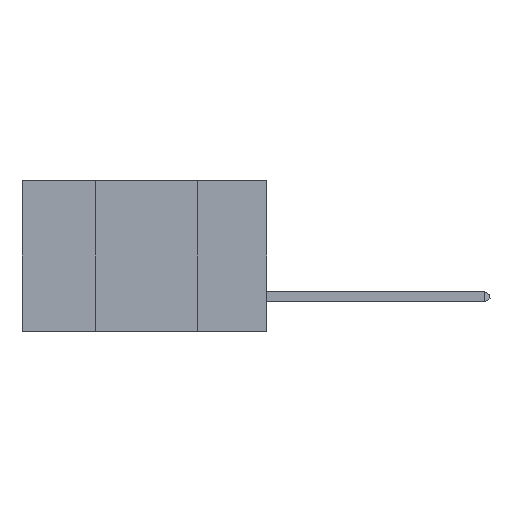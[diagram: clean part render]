
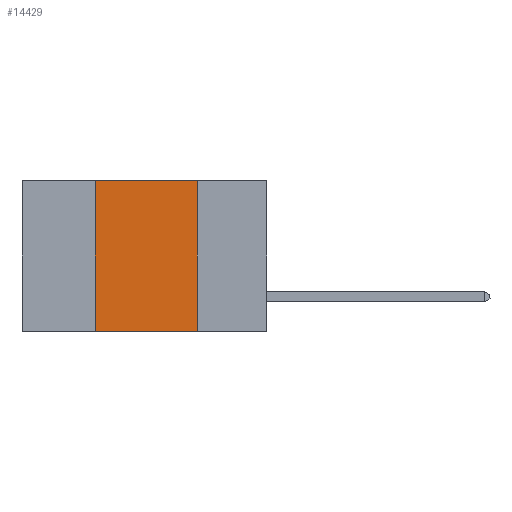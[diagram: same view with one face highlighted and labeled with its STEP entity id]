
A CAD part, left-side view. The second image highlights one B-rep face of the part: STEP entity #14429.
In plain terms, the highlighted planar face has unit normal (-1, 0, 0).
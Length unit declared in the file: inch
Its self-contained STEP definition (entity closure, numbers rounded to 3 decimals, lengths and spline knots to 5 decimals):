
#1192 = EDGE_CURVE ( 'NONE', #11467, #7550, #17679, .T. ) ;
#2617 = EDGE_CURVE ( 'NONE', #19219, #3082, #4087, .T. ) ;
#3082 = VERTEX_POINT ( 'NONE', #18073 ) ;
#3970 = ORIENTED_EDGE ( 'NONE', *, *, #1192, .F. ) ;
#4010 = ORIENTED_EDGE ( 'NONE', *, *, #2617, .F. ) ;
#4087 = LINE ( 'NONE', #20644, #19233 ) ;
#4941 = CARTESIAN_POINT ( 'NONE',  ( 0., 0.6, -0.37 ) ) ;
#5565 = EDGE_CURVE ( 'NONE', #3082, #11467, #14519, .T. ) ;
#7550 = VERTEX_POINT ( 'NONE', #15245 ) ;
#8149 = EDGE_CURVE ( 'NONE', #19219, #7550, #22864, .T. ) ;
#8182 = PLANE ( 'NONE',  #20640 ) ;
#8767 = DIRECTION ( 'NONE',  ( 0., -1., 0. ) ) ;
#10013 = ORIENTED_EDGE ( 'NONE', *, *, #5565, .F. ) ;
#11066 = FACE_OUTER_BOUND ( 'NONE', #22155, .T. ) ;
#11467 = VERTEX_POINT ( 'NONE', #24824 ) ;
#12265 = DIRECTION ( 'NONE',  ( 1., 0., 0. ) ) ;
#14363 = VECTOR ( 'NONE', #19330, 39.37008 ) ;
#14429 = ADVANCED_FACE ( 'NONE', ( #11066 ), #8182, .F. ) ;
#14519 = LINE ( 'NONE', #19071, #24931 ) ;
#15245 = CARTESIAN_POINT ( 'NONE',  ( 0., 0.17, -0.37 ) ) ;
#15873 = CARTESIAN_POINT ( 'NONE',  ( 0., 0.17, 0. ) ) ;
#16529 = DIRECTION ( 'NONE',  ( 0., 0., 1. ) ) ;
#17679 = LINE ( 'NONE', #15873, #26674 ) ;
#18073 = CARTESIAN_POINT ( 'NONE',  ( 0., 0.42, 0. ) ) ;
#19071 = CARTESIAN_POINT ( 'NONE',  ( 0., 0.6, 0. ) ) ;
#19219 = VERTEX_POINT ( 'NONE', #19747 ) ;
#19233 = VECTOR ( 'NONE', #16529, 39.37008 ) ;
#19330 = DIRECTION ( 'NONE',  ( 0., -1., 0. ) ) ;
#19747 = CARTESIAN_POINT ( 'NONE',  ( 0., 0.42, -0.37 ) ) ;
#20073 = DIRECTION ( 'NONE',  ( 0., 0., -1. ) ) ;
#20640 = AXIS2_PLACEMENT_3D ( 'NONE', #22656, #12265, #26719 ) ;
#20644 = CARTESIAN_POINT ( 'NONE',  ( 0., 0.42, 0. ) ) ;
#22155 = EDGE_LOOP ( 'NONE', ( #3970, #10013, #4010, #24350 ) ) ;
#22656 = CARTESIAN_POINT ( 'NONE',  ( 0., 0.6, 0. ) ) ;
#22864 = LINE ( 'NONE', #4941, #14363 ) ;
#24350 = ORIENTED_EDGE ( 'NONE', *, *, #8149, .T. ) ;
#24824 = CARTESIAN_POINT ( 'NONE',  ( 0., 0.17, 0. ) ) ;
#24931 = VECTOR ( 'NONE', #8767, 39.37008 ) ;
#26674 = VECTOR ( 'NONE', #20073, 39.37008 ) ;
#26719 = DIRECTION ( 'NONE',  ( 0., 0., -1. ) ) ;
